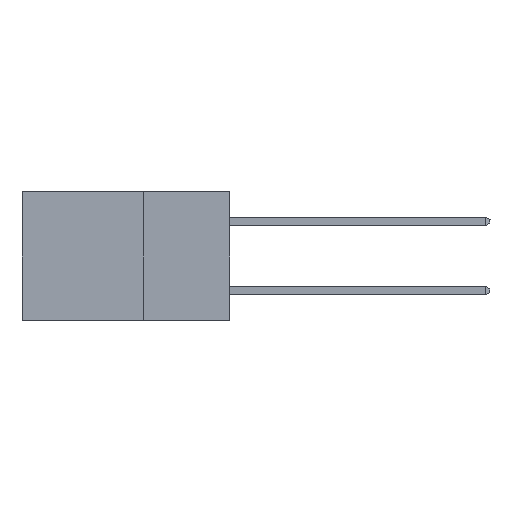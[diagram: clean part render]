
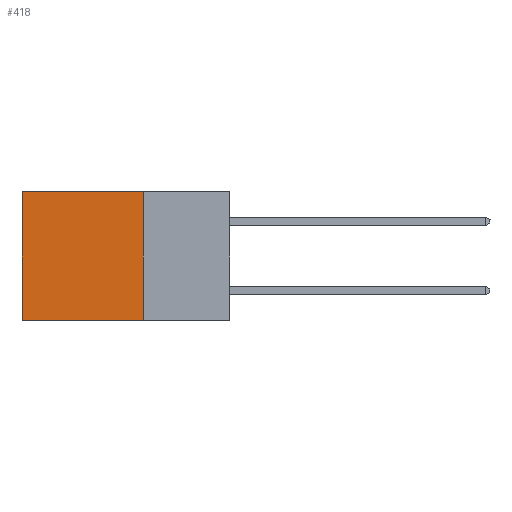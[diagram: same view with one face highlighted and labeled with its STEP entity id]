
A CAD part, left-side view. The second image highlights one B-rep face of the part: STEP entity #418.
In plain terms, the highlighted planar face has unit normal (-1, 0, 0).
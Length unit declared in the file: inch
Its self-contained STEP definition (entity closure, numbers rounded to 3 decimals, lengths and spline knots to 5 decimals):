
#418 = ADVANCED_FACE ( 'NONE', ( #2461 ), #6141, .F. ) ;
#608 = VECTOR ( 'NONE', #7542, 39.37008 ) ;
#636 = CARTESIAN_POINT ( 'NONE',  ( 0.2615, 0.6, -0.37 ) ) ;
#998 = ORIENTED_EDGE ( 'NONE', *, *, #1919, .T. ) ;
#1591 = VERTEX_POINT ( 'NONE', #8642 ) ;
#1919 = EDGE_CURVE ( 'NONE', #7287, #10912, #10080, .T. ) ;
#2273 = EDGE_CURVE ( 'NONE', #7811, #10912, #4562, .T. ) ;
#2461 = FACE_OUTER_BOUND ( 'NONE', #8945, .T. ) ;
#2673 = DIRECTION ( 'NONE',  ( 0., 0., -1. ) ) ;
#3025 = VECTOR ( 'NONE', #8891, 39.37008 ) ;
#3177 = CARTESIAN_POINT ( 'NONE',  ( 0.2615, 0.25, -0.37 ) ) ;
#3474 = AXIS2_PLACEMENT_3D ( 'NONE', #6927, #5917, #2673 ) ;
#4562 = LINE ( 'NONE', #8003, #6161 ) ;
#4934 = EDGE_CURVE ( 'NONE', #1591, #7287, #5427, .T. ) ;
#5160 = ORIENTED_EDGE ( 'NONE', *, *, #4934, .T. ) ;
#5427 = LINE ( 'NONE', #6948, #3025 ) ;
#5680 = DIRECTION ( 'NONE',  ( 0., 0., -1. ) ) ;
#5917 = DIRECTION ( 'NONE',  ( 1., 0., 0. ) ) ;
#6141 = PLANE ( 'NONE',  #3474 ) ;
#6161 = VECTOR ( 'NONE', #7139, 39.37008 ) ;
#6927 = CARTESIAN_POINT ( 'NONE',  ( 0.2615, 0.25, -0.37 ) ) ;
#6948 = CARTESIAN_POINT ( 'NONE',  ( 0.2615, 0.25, 0. ) ) ;
#7139 = DIRECTION ( 'NONE',  ( 0., 1., 0. ) ) ;
#7287 = VERTEX_POINT ( 'NONE', #9975 ) ;
#7542 = DIRECTION ( 'NONE',  ( 0., 0., -1. ) ) ;
#7811 = VERTEX_POINT ( 'NONE', #3177 ) ;
#8003 = CARTESIAN_POINT ( 'NONE',  ( 0.2615, 0.25, -0.37 ) ) ;
#8630 = ORIENTED_EDGE ( 'NONE', *, *, #2273, .F. ) ;
#8642 = CARTESIAN_POINT ( 'NONE',  ( 0.2615, 0.25, 0. ) ) ;
#8891 = DIRECTION ( 'NONE',  ( 0., 1., 0. ) ) ;
#8945 = EDGE_LOOP ( 'NONE', ( #998, #8630, #10599, #5160 ) ) ;
#9261 = CARTESIAN_POINT ( 'NONE',  ( 0.2615, 0.6, -0.37 ) ) ;
#9412 = LINE ( 'NONE', #10074, #608 ) ;
#9975 = CARTESIAN_POINT ( 'NONE',  ( 0.2615, 0.6, 0. ) ) ;
#10074 = CARTESIAN_POINT ( 'NONE',  ( 0.2615, 0.25, -0.37 ) ) ;
#10080 = LINE ( 'NONE', #9261, #10855 ) ;
#10556 = EDGE_CURVE ( 'NONE', #1591, #7811, #9412, .T. ) ;
#10599 = ORIENTED_EDGE ( 'NONE', *, *, #10556, .F. ) ;
#10855 = VECTOR ( 'NONE', #5680, 39.37008 ) ;
#10912 = VERTEX_POINT ( 'NONE', #636 ) ;
